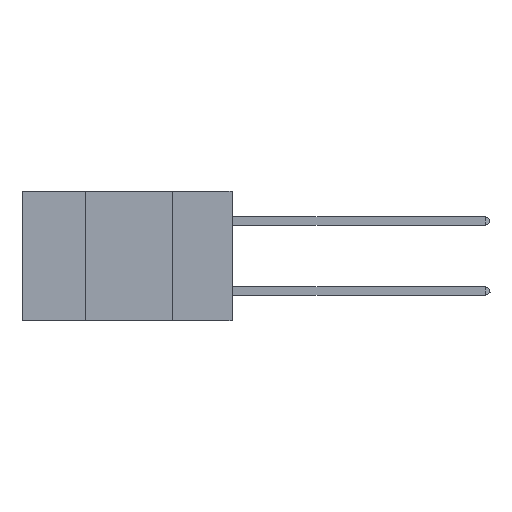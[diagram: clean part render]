
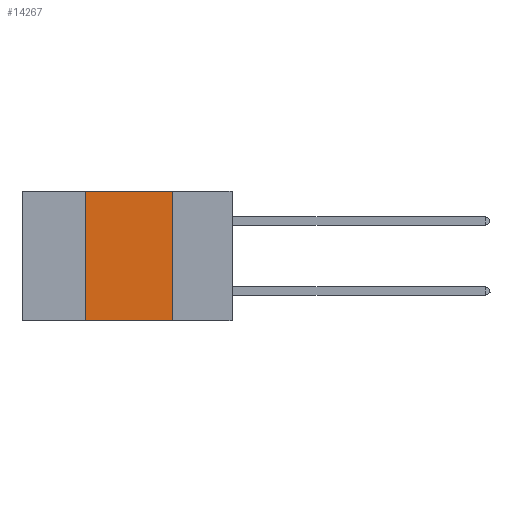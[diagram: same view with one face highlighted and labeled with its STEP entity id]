
A CAD part, left-side view. The second image highlights one B-rep face of the part: STEP entity #14267.
In plain terms, the highlighted planar face has unit normal (-1, 0, 0).
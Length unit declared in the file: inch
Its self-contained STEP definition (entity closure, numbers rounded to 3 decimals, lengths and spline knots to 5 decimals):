
#2835 = ORIENTED_EDGE ( 'NONE', *, *, #25289, .F. ) ;
#3479 = CARTESIAN_POINT ( 'NONE',  ( 0., 0.42, 0. ) ) ;
#3584 = DIRECTION ( 'NONE',  ( 0., -1., 0. ) ) ;
#4592 = CARTESIAN_POINT ( 'NONE',  ( 0., 0.17, 0. ) ) ;
#5193 = ORIENTED_EDGE ( 'NONE', *, *, #18189, .T. ) ;
#8628 = DIRECTION ( 'NONE',  ( 0., 0., 1. ) ) ;
#9505 = VERTEX_POINT ( 'NONE', #14867 ) ;
#9847 = VECTOR ( 'NONE', #21652, 39.37008 ) ;
#10894 = ORIENTED_EDGE ( 'NONE', *, *, #25379, .F. ) ;
#11399 = LINE ( 'NONE', #3479, #15919 ) ;
#11516 = DIRECTION ( 'NONE',  ( 0., -1., 0. ) ) ;
#11775 = VECTOR ( 'NONE', #3584, 39.37008 ) ;
#12284 = CARTESIAN_POINT ( 'NONE',  ( 0., 0.17, 0. ) ) ;
#12566 = VERTEX_POINT ( 'NONE', #28367 ) ;
#13855 = EDGE_LOOP ( 'NONE', ( #29568, #2835, #10894, #5193 ) ) ;
#14267 = ADVANCED_FACE ( 'NONE', ( #17038 ), #30070, .F. ) ;
#14867 = CARTESIAN_POINT ( 'NONE',  ( 0., 0.42, -0.37 ) ) ;
#15919 = VECTOR ( 'NONE', #8628, 39.37008 ) ;
#16615 = LINE ( 'NONE', #4592, #9847 ) ;
#16894 = CARTESIAN_POINT ( 'NONE',  ( 0., 0.17, -0.37 ) ) ;
#17038 = FACE_OUTER_BOUND ( 'NONE', #13855, .T. ) ;
#17319 = EDGE_CURVE ( 'NONE', #23025, #27747, #16615, .T. ) ;
#17993 = CARTESIAN_POINT ( 'NONE',  ( 0., 0.6, 0. ) ) ;
#18189 = EDGE_CURVE ( 'NONE', #9505, #27747, #19996, .T. ) ;
#19996 = LINE ( 'NONE', #28095, #26409 ) ;
#20681 = DIRECTION ( 'NONE',  ( 1., 0., 0. ) ) ;
#21652 = DIRECTION ( 'NONE',  ( 0., 0., -1. ) ) ;
#22356 = LINE ( 'NONE', #25380, #11775 ) ;
#23025 = VERTEX_POINT ( 'NONE', #12284 ) ;
#23921 = AXIS2_PLACEMENT_3D ( 'NONE', #17993, #20681, #27946 ) ;
#25289 = EDGE_CURVE ( 'NONE', #12566, #23025, #22356, .T. ) ;
#25379 = EDGE_CURVE ( 'NONE', #9505, #12566, #11399, .T. ) ;
#25380 = CARTESIAN_POINT ( 'NONE',  ( 0., 0.6, 0. ) ) ;
#26409 = VECTOR ( 'NONE', #11516, 39.37008 ) ;
#27747 = VERTEX_POINT ( 'NONE', #16894 ) ;
#27946 = DIRECTION ( 'NONE',  ( 0., 0., -1. ) ) ;
#28095 = CARTESIAN_POINT ( 'NONE',  ( 0., 0.6, -0.37 ) ) ;
#28367 = CARTESIAN_POINT ( 'NONE',  ( 0., 0.42, 0. ) ) ;
#29568 = ORIENTED_EDGE ( 'NONE', *, *, #17319, .F. ) ;
#30070 = PLANE ( 'NONE',  #23921 ) ;
